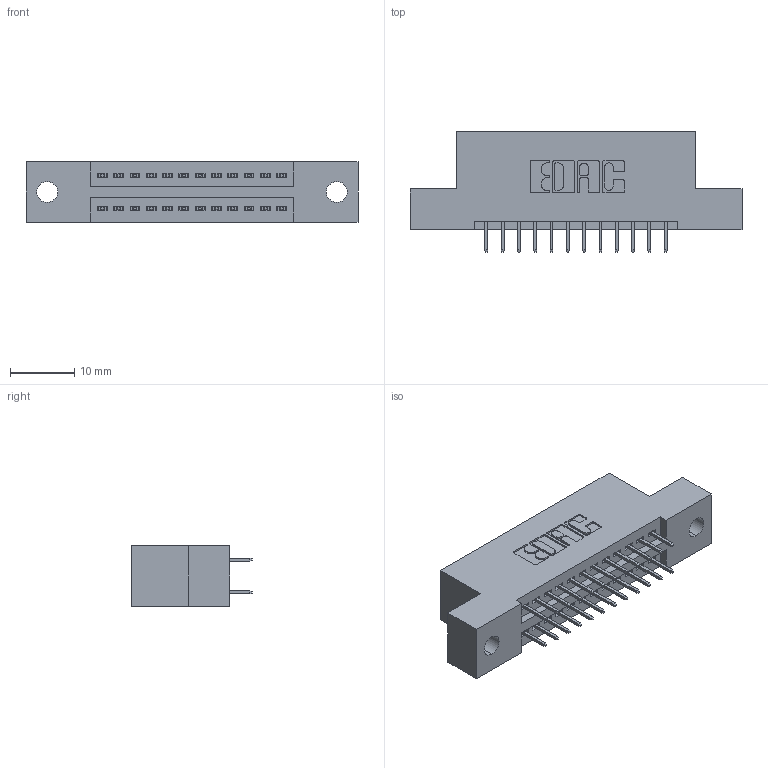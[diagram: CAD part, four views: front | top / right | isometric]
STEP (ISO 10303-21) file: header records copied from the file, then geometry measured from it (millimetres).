
FILE_DESCRIPTION (( 'STEP AP203' ), '1' );
FILE_NAME ('845-024-525-202.STEP', '2020-09-22T21:32:40', ( '' ), ( '' ), 'SwSTEP 2.0', 'SolidWorks 2020', '' );
FILE_SCHEMA (( 'CONFIG_CONTROL_DESIGN' ));
Length unit declared in the file: inch
Products named in the file (3): 845-024-525-202; 845 Part_Flush Mounting Lugs - 0.128 Dia; 345-292-001_345-293-125
Assembly tree (25 placements, depth 2):
  845-024-525-202
    845 Part_Flush Mounting Lugs - 0.128 Dia
    345-292-001_345-293-125  x24
Bounding box: 51.69 x 18.72 x 9.4 mm (x, y, z)
Volume: 4666.5 mm3; surface area: 5925 mm2
Topology: 25 solids, 25 shells, 1422 faces, 4013 edges, 2578 vertices
Faces by surface type: plane 1016, cylinder 406
Entity records: 13531 total; most frequent: CARTESIAN_POINT 2296, ORIENTED_EDGE 2230, DIRECTION 2063, EDGE_CURVE 1115, VECTOR 939, LINE 939, VERTEX_POINT 738, AXIS2_PLACEMENT_3D 562
